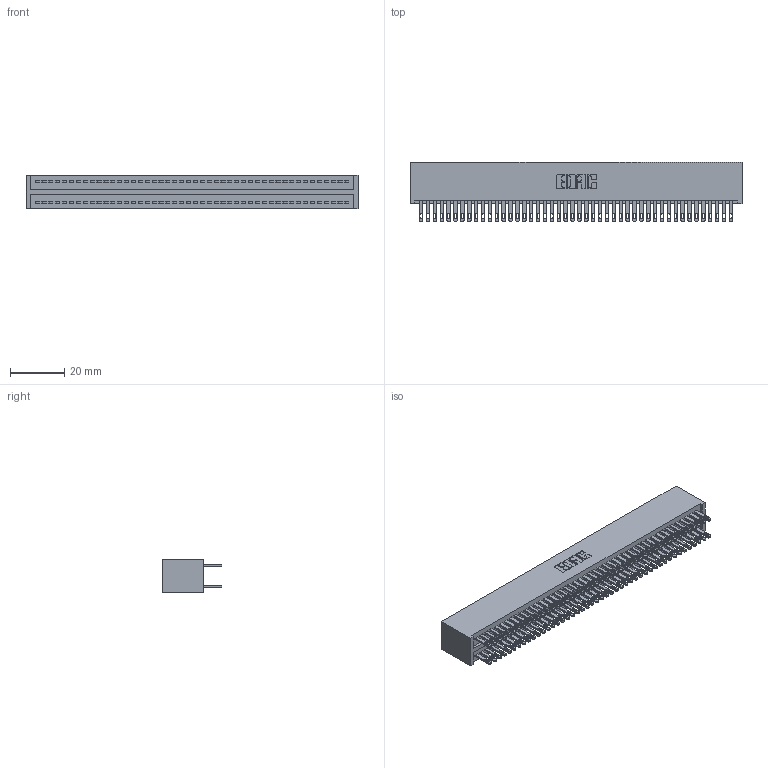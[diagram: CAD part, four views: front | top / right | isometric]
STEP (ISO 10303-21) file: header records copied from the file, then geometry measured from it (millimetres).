
FILE_DESCRIPTION (( 'STEP AP203' ), '1' );
FILE_NAME ('325-092-500-201.STEP', '2020-02-25T05:44:29', ( '' ), ( '' ), 'SwSTEP 2.0', 'SolidWorks 2016', '' );
FILE_SCHEMA (( 'CONFIG_CONTROL_DESIGN' ));
Length unit declared in the file: inch
Products named in the file (3): 325-292-001_325-293-100; 325-092-500-201; 325 Part_Lugless
Assembly tree (93 placements, depth 2):
  325-092-500-201
    325 Part_Lugless
    325-292-001_325-293-100  x92
Bounding box: 122.48 x 21.84 x 12.45 mm (x, y, z)
Volume: 16734.7 mm3; surface area: 21973 mm2
Topology: 93 solids, 93 shells, 4522 faces, 13811 edges, 9206 vertices
Faces by surface type: plane 2826, cylinder 1696
Entity records: 28729 total; most frequent: CARTESIAN_POINT 4754, ORIENTED_EDGE 4690, DIRECTION 4049, EDGE_CURVE 2345, LINE 2221, VECTOR 2221, VERTEX_POINT 1562, AXIS2_PLACEMENT_3D 914
